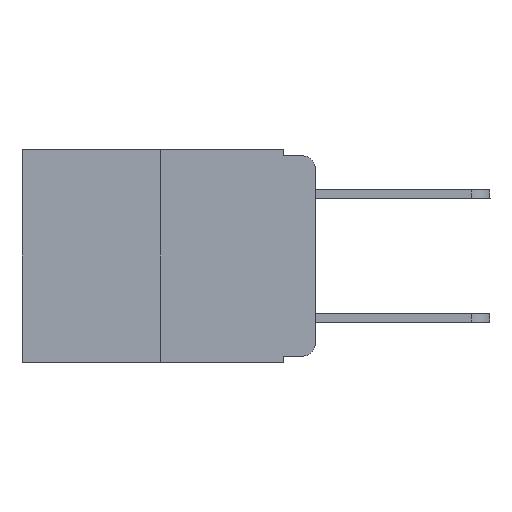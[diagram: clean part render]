
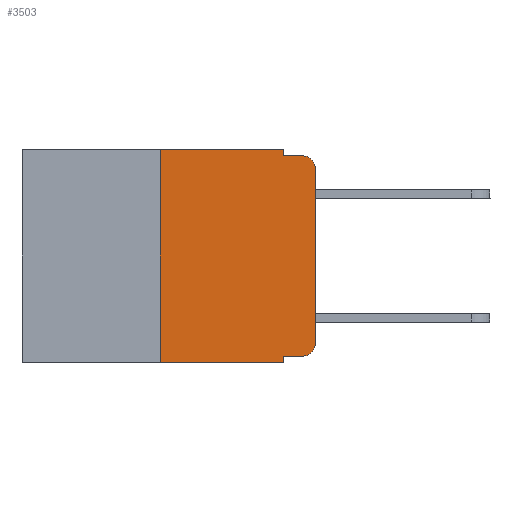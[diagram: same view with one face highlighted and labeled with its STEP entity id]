
A CAD part, left-side view. The second image highlights one B-rep face of the part: STEP entity #3503.
In plain terms, the highlighted planar face has unit normal (-1, 0, 0).
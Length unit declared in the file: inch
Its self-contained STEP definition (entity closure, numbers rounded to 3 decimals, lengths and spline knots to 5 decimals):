
#101 = VERTEX_POINT ( 'NONE', #7219 ) ;
#127 = EDGE_CURVE ( 'NONE', #3638, #10667, #11203, .T. ) ;
#292 = AXIS2_PLACEMENT_3D ( 'NONE', #5503, #10657, #10403 ) ;
#357 = EDGE_CURVE ( 'NONE', #7543, #101, #14866, .T. ) ;
#1070 = EDGE_LOOP ( 'NONE', ( #6149, #10742, #10147, #8812, #6982, #11055, #6499, #9944, #5213, #12976 ) ) ;
#1463 = CARTESIAN_POINT ( 'NONE',  ( 0., 0.051, -0.343 ) ) ;
#2056 = CARTESIAN_POINT ( 'NONE',  ( 0., 0.25, 0. ) ) ;
#2238 = DIRECTION ( 'NONE',  ( 0., -1., 0. ) ) ;
#2511 = VERTEX_POINT ( 'NONE', #9010 ) ;
#2577 = VECTOR ( 'NONE', #7192, 39.37008 ) ;
#2793 = EDGE_CURVE ( 'NONE', #10056, #2883, #8656, .T. ) ;
#2796 = VECTOR ( 'NONE', #15949, 39.37008 ) ;
#2883 = VERTEX_POINT ( 'NONE', #6120 ) ;
#3030 = VECTOR ( 'NONE', #2238, 39.37008 ) ;
#3083 = VECTOR ( 'NONE', #11277, 39.37008 ) ;
#3155 = DIRECTION ( 'NONE',  ( 0., 0., -1. ) ) ;
#3332 = CARTESIAN_POINT ( 'NONE',  ( 0., 0.473, 0. ) ) ;
#3503 = ADVANCED_FACE ( 'NONE', ( #4637 ), #8362, .F. ) ;
#3551 = AXIS2_PLACEMENT_3D ( 'NONE', #5618, #4425, #9488 ) ;
#3638 = VERTEX_POINT ( 'NONE', #8018 ) ;
#4328 = VECTOR ( 'NONE', #6556, 39.37008 ) ;
#4425 = DIRECTION ( 'NONE',  ( -1., 0., 0. ) ) ;
#4637 = FACE_OUTER_BOUND ( 'NONE', #1070, .T. ) ;
#5040 = LINE ( 'NONE', #15497, #8798 ) ;
#5213 = ORIENTED_EDGE ( 'NONE', *, *, #127, .T. ) ;
#5503 = CARTESIAN_POINT ( 'NONE',  ( 0., 0.02, -0.313 ) ) ;
#5618 = CARTESIAN_POINT ( 'NONE',  ( 0., 0.02, -0.03 ) ) ;
#5661 = LINE ( 'NONE', #10815, #2796 ) ;
#5751 = AXIS2_PLACEMENT_3D ( 'NONE', #12082, #5834, #10984 ) ;
#5834 = DIRECTION ( 'NONE',  ( 1., 0., 0. ) ) ;
#6120 = CARTESIAN_POINT ( 'NONE',  ( 0., 0.02, -0.01 ) ) ;
#6149 = ORIENTED_EDGE ( 'NONE', *, *, #12638, .T. ) ;
#6206 = EDGE_CURVE ( 'NONE', #3638, #12406, #7190, .T. ) ;
#6499 = ORIENTED_EDGE ( 'NONE', *, *, #13689, .T. ) ;
#6556 = DIRECTION ( 'NONE',  ( 0., 0., -1. ) ) ;
#6982 = ORIENTED_EDGE ( 'NONE', *, *, #357, .F. ) ;
#7107 = CARTESIAN_POINT ( 'NONE',  ( 0., 0.051, 0. ) ) ;
#7108 = LINE ( 'NONE', #8153, #2577 ) ;
#7190 = LINE ( 'NONE', #7107, #13421 ) ;
#7192 = DIRECTION ( 'NONE',  ( 0., -1., 0. ) ) ;
#7198 = DIRECTION ( 'NONE',  ( 0., -1., 0. ) ) ;
#7219 = CARTESIAN_POINT ( 'NONE',  ( 0., 0.051, 0. ) ) ;
#7543 = VERTEX_POINT ( 'NONE', #2056 ) ;
#7832 = EDGE_CURVE ( 'NONE', #10667, #2511, #15362, .T. ) ;
#7883 = VECTOR ( 'NONE', #7198, 39.37008 ) ;
#7972 = CARTESIAN_POINT ( 'NONE',  ( 0., 0.02, -0.333 ) ) ;
#8018 = CARTESIAN_POINT ( 'NONE',  ( 0., 0.051, -0.333 ) ) ;
#8153 = CARTESIAN_POINT ( 'NONE',  ( 0., 0.051, -0.01 ) ) ;
#8261 = VERTEX_POINT ( 'NONE', #10142 ) ;
#8362 = PLANE ( 'NONE',  #5751 ) ;
#8656 = CIRCLE ( 'NONE', #3551, 0.02 ) ;
#8792 = EDGE_CURVE ( 'NONE', #101, #8261, #9246, .T. ) ;
#8798 = VECTOR ( 'NONE', #14221, 39.37008 ) ;
#8812 = ORIENTED_EDGE ( 'NONE', *, *, #8792, .F. ) ;
#9010 = CARTESIAN_POINT ( 'NONE',  ( 0., 0., -0.313 ) ) ;
#9246 = LINE ( 'NONE', #14400, #4328 ) ;
#9488 = DIRECTION ( 'NONE',  ( 0., 0., -1. ) ) ;
#9743 = CARTESIAN_POINT ( 'NONE',  ( 0., 0., -0.03 ) ) ;
#9944 = ORIENTED_EDGE ( 'NONE', *, *, #6206, .F. ) ;
#10056 = VERTEX_POINT ( 'NONE', #9743 ) ;
#10142 = CARTESIAN_POINT ( 'NONE',  ( 0., 0.051, -0.01 ) ) ;
#10147 = ORIENTED_EDGE ( 'NONE', *, *, #13966, .F. ) ;
#10403 = DIRECTION ( 'NONE',  ( 0., 0., -1. ) ) ;
#10657 = DIRECTION ( 'NONE',  ( -1., 0., 0. ) ) ;
#10667 = VERTEX_POINT ( 'NONE', #7972 ) ;
#10742 = ORIENTED_EDGE ( 'NONE', *, *, #2793, .T. ) ;
#10815 = CARTESIAN_POINT ( 'NONE',  ( 0., 0., 0. ) ) ;
#10984 = DIRECTION ( 'NONE',  ( 0., 0., -1. ) ) ;
#11055 = ORIENTED_EDGE ( 'NONE', *, *, #15900, .F. ) ;
#11203 = LINE ( 'NONE', #13792, #3030 ) ;
#11229 = VERTEX_POINT ( 'NONE', #15868 ) ;
#11277 = DIRECTION ( 'NONE',  ( 0., -1., 0. ) ) ;
#12082 = CARTESIAN_POINT ( 'NONE',  ( 0., 0.473, 0. ) ) ;
#12406 = VERTEX_POINT ( 'NONE', #1463 ) ;
#12638 = EDGE_CURVE ( 'NONE', #2511, #10056, #5661, .T. ) ;
#12976 = ORIENTED_EDGE ( 'NONE', *, *, #7832, .T. ) ;
#13421 = VECTOR ( 'NONE', #3155, 39.37008 ) ;
#13689 = EDGE_CURVE ( 'NONE', #11229, #12406, #13964, .T. ) ;
#13792 = CARTESIAN_POINT ( 'NONE',  ( 0., 0.051, -0.333 ) ) ;
#13964 = LINE ( 'NONE', #16411, #3083 ) ;
#13966 = EDGE_CURVE ( 'NONE', #8261, #2883, #7108, .T. ) ;
#14221 = DIRECTION ( 'NONE',  ( 0., 0., 1. ) ) ;
#14400 = CARTESIAN_POINT ( 'NONE',  ( 0., 0.051, 0. ) ) ;
#14866 = LINE ( 'NONE', #3332, #7883 ) ;
#15362 = CIRCLE ( 'NONE', #292, 0.02 ) ;
#15497 = CARTESIAN_POINT ( 'NONE',  ( 0., 0.25, 0. ) ) ;
#15868 = CARTESIAN_POINT ( 'NONE',  ( 0., 0.25, -0.343 ) ) ;
#15900 = EDGE_CURVE ( 'NONE', #11229, #7543, #5040, .T. ) ;
#15949 = DIRECTION ( 'NONE',  ( 0., 0., 1. ) ) ;
#16411 = CARTESIAN_POINT ( 'NONE',  ( 0., 0.473, -0.343 ) ) ;
